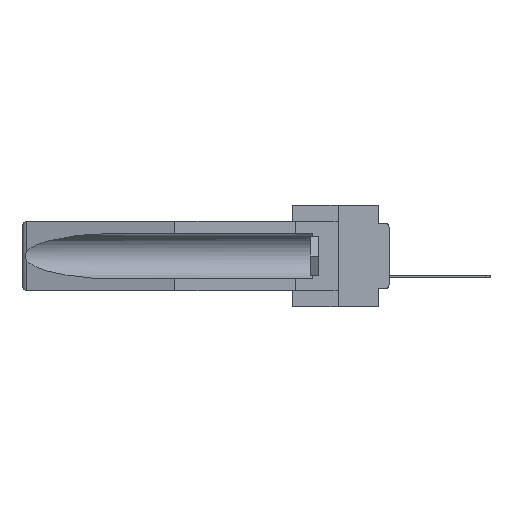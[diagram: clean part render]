
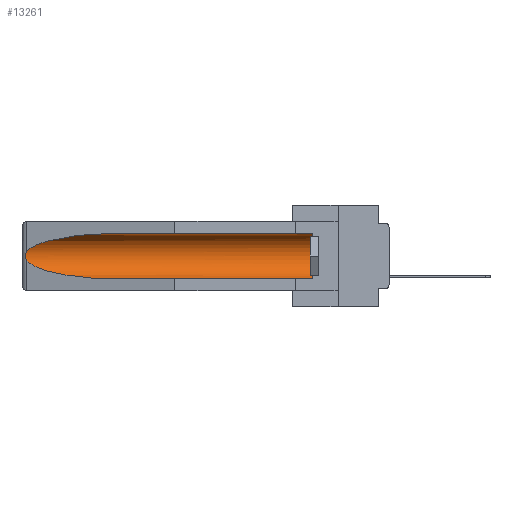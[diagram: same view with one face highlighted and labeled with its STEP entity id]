
A CAD part, left-side view. The second image highlights one B-rep face of the part: STEP entity #13261.
In plain terms, the highlighted cylindrical face has radius 2.857 mm (diameter 5.715 mm), a partial arc.
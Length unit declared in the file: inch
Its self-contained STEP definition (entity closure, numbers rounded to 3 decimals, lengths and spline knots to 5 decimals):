
#35 = EDGE_LOOP ( 'NONE', ( #11078, #24717, #11580, #23357, #5958, #2381 ) ) ;
#2381 = ORIENTED_EDGE ( 'NONE', *, *, #5790, .T. ) ;
#2474 = DIRECTION ( 'NONE',  ( 0., 1., 0. ) ) ;
#2868 = CYLINDRICAL_SURFACE ( 'NONE', #19861, 0.1125 ) ;
#2876 = EDGE_CURVE ( 'NONE', #15573, #17908, #26018, .T. ) ;
#4847 = LINE ( 'NONE', #15523, #16761 ) ;
#5239 = CARTESIAN_POINT ( 'NONE',  ( 0.25451, 1.48313, -0.24835 ) ) ;
#5787 = DIRECTION ( 'NONE',  ( 0., 1., 0. ) ) ;
#5790 = EDGE_CURVE ( 'NONE', #22206, #8447, #4847, .T. ) ;
#5874 = VECTOR ( 'NONE', #8115, 39.37008 ) ;
#5958 = ORIENTED_EDGE ( 'NONE', *, *, #11647, .T. ) ;
#6155 = VERTEX_POINT ( 'NONE', #27990 ) ;
#6263 = CARTESIAN_POINT ( 'NONE',  ( 0.155, -0.30754, -0.1715 ) ) ;
#6422 = CARTESIAN_POINT ( 'NONE',  ( 0.26537, 1.52718, -0.14972 ) ) ;
#6907 = EDGE_CURVE ( 'NONE', #6155, #17908, #11752, .T. ) ;
#7161 = DIRECTION ( 'NONE',  ( 0., 0., 1. ) ) ;
#7679 = CARTESIAN_POINT ( 'NONE',  ( 0.26537, 1.52718, -0.19328 ) ) ;
#7783 = CARTESIAN_POINT ( 'NONE',  ( 0.21114, 1.30732, -0.284 ) ) ;
#8115 = DIRECTION ( 'NONE',  ( 0., 1., 0. ) ) ;
#8233 = AXIS2_PLACEMENT_3D ( 'NONE', #21623, #28253, #15355 ) ;
#8447 = VERTEX_POINT ( 'NONE', #16377 ) ;
#8660 = CARTESIAN_POINT ( 'NONE',  ( 0.2675, 1.53308, -0.17534 ) ) ;
#8877 = CARTESIAN_POINT ( 'NONE',  ( 0.21114, 1.30732, -0.059 ) ) ;
#8953 = CIRCLE ( 'NONE', #8233, 0.1125 ) ;
#9205 =( BOUNDED_CURVE ( )  B_SPLINE_CURVE ( 3, ( #15724, #8877, #22274, #13365 ),
 .UNSPECIFIED., .F., .F. ) 
 B_SPLINE_CURVE_WITH_KNOTS ( ( 4, 4 ),
 ( 4.71239, 6.08839 ),
 .UNSPECIFIED. ) 
 CURVE ( )  GEOMETRIC_REPRESENTATION_ITEM ( )  RATIONAL_B_SPLINE_CURVE ( ( 1., 0.848, 0.848, 1. ) ) 
 REPRESENTATION_ITEM ( '' )  );
#10908 = EDGE_CURVE ( 'NONE', #27694, #15573, #15676, .T. ) ;
#11078 = ORIENTED_EDGE ( 'NONE', *, *, #16048, .T. ) ;
#11580 = ORIENTED_EDGE ( 'NONE', *, *, #2876, .T. ) ;
#11647 = EDGE_CURVE ( 'NONE', #6155, #22206, #8953, .T. ) ;
#11752 = LINE ( 'NONE', #20790, #5874 ) ;
#12691 = FACE_OUTER_BOUND ( 'NONE', #35, .T. ) ;
#13062 = CARTESIAN_POINT ( 'NONE',  ( 0.26654, 1.53092, -0.15636 ) ) ;
#13261 = ADVANCED_FACE ( 'NONE', ( #12691 ), #2868, .F. ) ;
#13365 = CARTESIAN_POINT ( 'NONE',  ( 0.26537, 1.52718, -0.14972 ) ) ;
#14939 = CARTESIAN_POINT ( 'NONE',  ( 0.26537, 1.52718, -0.19328 ) ) ;
#15355 = DIRECTION ( 'NONE',  ( 0., 0., 1. ) ) ;
#15523 = CARTESIAN_POINT ( 'NONE',  ( 0.155, -0.30754, -0.059 ) ) ;
#15573 = VERTEX_POINT ( 'NONE', #18456 ) ;
#15676 = B_SPLINE_CURVE_WITH_KNOTS ( 'NONE', 3,
 ( #6422, #19621, #13062, #17175, #26199, #8660, #21683, #24263, #26010, #14939 ),
 .UNSPECIFIED., .F., .F.,
 ( 4, 2, 2, 2, 4 ),
 ( 0., 0.00029, 0.00058, 0.00087, 0.00117 ),
 .UNSPECIFIED. ) ;
#15724 = CARTESIAN_POINT ( 'NONE',  ( 0.155, 1.07973, -0.059 ) ) ;
#16048 = EDGE_CURVE ( 'NONE', #8447, #27694, #9205, .T. ) ;
#16377 = CARTESIAN_POINT ( 'NONE',  ( 0.155, 1.07973, -0.059 ) ) ;
#16420 = CARTESIAN_POINT ( 'NONE',  ( 0.26537, 1.52718, -0.14972 ) ) ;
#16761 = VECTOR ( 'NONE', #2474, 39.37008 ) ;
#17175 = CARTESIAN_POINT ( 'NONE',  ( 0.2673, 1.5327, -0.16383 ) ) ;
#17908 = VERTEX_POINT ( 'NONE', #22559 ) ;
#18456 = CARTESIAN_POINT ( 'NONE',  ( 0.26537, 1.52718, -0.19328 ) ) ;
#19621 = CARTESIAN_POINT ( 'NONE',  ( 0.26597, 1.52961, -0.15275 ) ) ;
#19861 = AXIS2_PLACEMENT_3D ( 'NONE', #6263, #5787, #7161 ) ;
#19897 = CARTESIAN_POINT ( 'NONE',  ( 0.155, 0.126, -0.059 ) ) ;
#20790 = CARTESIAN_POINT ( 'NONE',  ( 0.155, -0.30754, -0.284 ) ) ;
#21623 = CARTESIAN_POINT ( 'NONE',  ( 0.155, 0.126, -0.1715 ) ) ;
#21683 = CARTESIAN_POINT ( 'NONE',  ( 0.2673, 1.53269, -0.17917 ) ) ;
#22206 = VERTEX_POINT ( 'NONE', #19897 ) ;
#22274 = CARTESIAN_POINT ( 'NONE',  ( 0.25451, 1.48313, -0.09465 ) ) ;
#22559 = CARTESIAN_POINT ( 'NONE',  ( 0.155, 1.07973, -0.284 ) ) ;
#23357 = ORIENTED_EDGE ( 'NONE', *, *, #6907, .F. ) ;
#24263 = CARTESIAN_POINT ( 'NONE',  ( 0.26655, 1.53094, -0.18657 ) ) ;
#24717 = ORIENTED_EDGE ( 'NONE', *, *, #10908, .T. ) ;
#26010 = CARTESIAN_POINT ( 'NONE',  ( 0.26597, 1.5296, -0.19026 ) ) ;
#26018 =( BOUNDED_CURVE ( )  B_SPLINE_CURVE ( 3, ( #7679, #5239, #7783, #27706 ),
 .UNSPECIFIED., .F., .F. ) 
 B_SPLINE_CURVE_WITH_KNOTS ( ( 4, 4 ),
 ( 0.1948, 1.5708 ),
 .UNSPECIFIED. ) 
 CURVE ( )  GEOMETRIC_REPRESENTATION_ITEM ( )  RATIONAL_B_SPLINE_CURVE ( ( 1., 0.848, 0.848, 1. ) ) 
 REPRESENTATION_ITEM ( '' )  );
#26199 = CARTESIAN_POINT ( 'NONE',  ( 0.2675, 1.53308, -0.16763 ) ) ;
#27694 = VERTEX_POINT ( 'NONE', #16420 ) ;
#27706 = CARTESIAN_POINT ( 'NONE',  ( 0.155, 1.07973, -0.284 ) ) ;
#27990 = CARTESIAN_POINT ( 'NONE',  ( 0.155, 0.126, -0.284 ) ) ;
#28253 = DIRECTION ( 'NONE',  ( 0., -1., 0. ) ) ;
